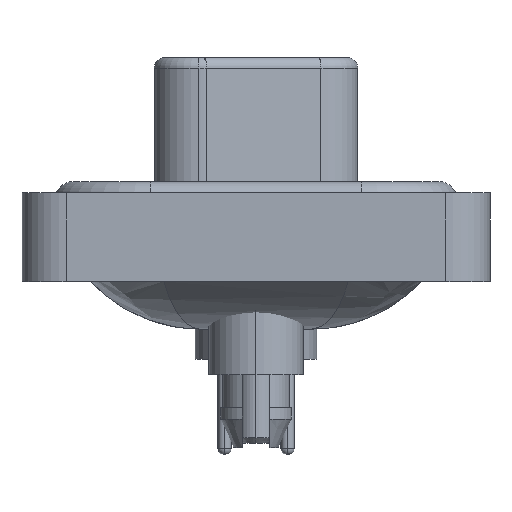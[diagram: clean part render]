
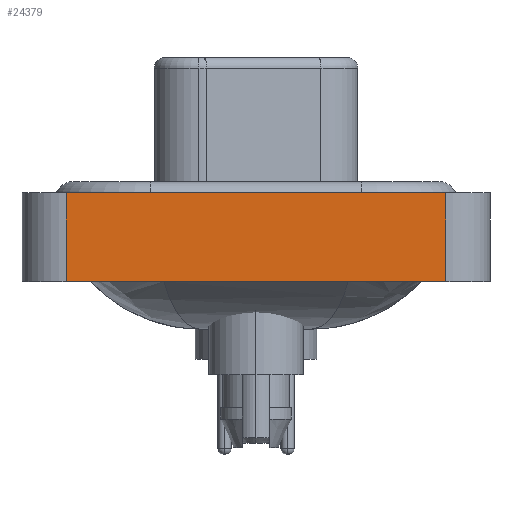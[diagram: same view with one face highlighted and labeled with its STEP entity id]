
A CAD part, left-side view. The second image highlights one B-rep face of the part: STEP entity #24379.
In plain terms, the highlighted planar face has unit normal (-1, 0, 0).
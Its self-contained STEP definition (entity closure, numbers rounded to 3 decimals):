
#524 = PLANE ( 'NONE',  #925 ) ;
#925 = AXIS2_PLACEMENT_3D ( 'NONE', #24380, #14490, #22543 ) ;
#1124 = LINE ( 'NONE', #20559, #3041 ) ;
#2159 = CARTESIAN_POINT ( 'NONE',  ( -7.35, 8.55, 0.4 ) ) ;
#2750 = VECTOR ( 'NONE', #2995, 1000. ) ;
#2995 = DIRECTION ( 'NONE',  ( 0., -1., 0. ) ) ;
#3041 = VECTOR ( 'NONE', #16893, 1000. ) ;
#3723 = CARTESIAN_POINT ( 'NONE',  ( -7.35, -8.55, -3.6 ) ) ;
#3796 = CARTESIAN_POINT ( 'NONE',  ( -7.35, -8.55, -3.6 ) ) ;
#5192 = EDGE_CURVE ( 'NONE', #19530, #18826, #21647, .T. ) ;
#6123 = DIRECTION ( 'NONE',  ( 0., -1., 0. ) ) ;
#6428 = EDGE_CURVE ( 'NONE', #16874, #19530, #10680, .T. ) ;
#7708 = VERTEX_POINT ( 'NONE', #2159 ) ;
#10680 = LINE ( 'NONE', #24753, #2750 ) ;
#11120 = ORIENTED_EDGE ( 'NONE', *, *, #5192, .T. ) ;
#12637 = VECTOR ( 'NONE', #22279, 1000. ) ;
#13296 = EDGE_CURVE ( 'NONE', #16874, #7708, #1124, .T. ) ;
#13863 = LINE ( 'NONE', #16066, #24515 ) ;
#14010 = EDGE_CURVE ( 'NONE', #7708, #18826, #13863, .T. ) ;
#14490 = DIRECTION ( 'NONE',  ( -1., 0., 0. ) ) ;
#14669 = ORIENTED_EDGE ( 'NONE', *, *, #14010, .F. ) ;
#16066 = CARTESIAN_POINT ( 'NONE',  ( -7.35, -8.55, 0.4 ) ) ;
#16812 = ORIENTED_EDGE ( 'NONE', *, *, #13296, .F. ) ;
#16874 = VERTEX_POINT ( 'NONE', #18775 ) ;
#16893 = DIRECTION ( 'NONE',  ( 0., 0., 1. ) ) ;
#17155 = ORIENTED_EDGE ( 'NONE', *, *, #6428, .T. ) ;
#18389 = FACE_OUTER_BOUND ( 'NONE', #20294, .T. ) ;
#18775 = CARTESIAN_POINT ( 'NONE',  ( -7.35, 8.55, -3.6 ) ) ;
#18826 = VERTEX_POINT ( 'NONE', #24288 ) ;
#19530 = VERTEX_POINT ( 'NONE', #3723 ) ;
#20294 = EDGE_LOOP ( 'NONE', ( #11120, #14669, #16812, #17155 ) ) ;
#20559 = CARTESIAN_POINT ( 'NONE',  ( -7.35, 8.55, -3.6 ) ) ;
#21647 = LINE ( 'NONE', #3796, #12637 ) ;
#22279 = DIRECTION ( 'NONE',  ( 0., 0., 1. ) ) ;
#22543 = DIRECTION ( 'NONE',  ( 0., 0., 1. ) ) ;
#24288 = CARTESIAN_POINT ( 'NONE',  ( -7.35, -8.55, 0.4 ) ) ;
#24379 = ADVANCED_FACE ( 'NONE', ( #18389 ), #524, .T. ) ;
#24380 = CARTESIAN_POINT ( 'NONE',  ( -7.35, -8.55, -3.6 ) ) ;
#24515 = VECTOR ( 'NONE', #6123, 1000. ) ;
#24753 = CARTESIAN_POINT ( 'NONE',  ( -7.35, -8.55, -3.6 ) ) ;
